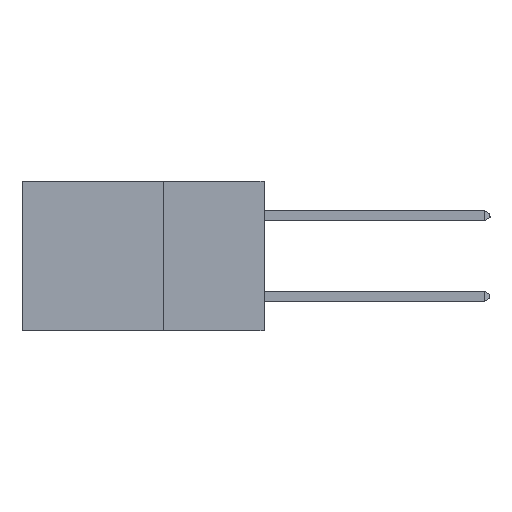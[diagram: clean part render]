
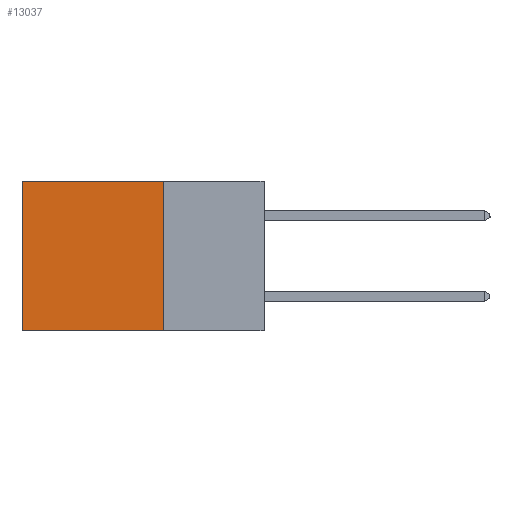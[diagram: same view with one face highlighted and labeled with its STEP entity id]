
A CAD part, left-side view. The second image highlights one B-rep face of the part: STEP entity #13037.
In plain terms, the highlighted planar face has unit normal (-1, 0, 0).
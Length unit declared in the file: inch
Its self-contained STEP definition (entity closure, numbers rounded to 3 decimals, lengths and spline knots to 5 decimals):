
#670 = AXIS2_PLACEMENT_3D ( 'NONE', #2234, #16523, #4302 ) ;
#1079 = CARTESIAN_POINT ( 'NONE',  ( 0.298, 0.6, -0.37 ) ) ;
#1245 = CARTESIAN_POINT ( 'NONE',  ( 0.298, 0.25, 0. ) ) ;
#2234 = CARTESIAN_POINT ( 'NONE',  ( 0.298, 0.25, 0. ) ) ;
#2896 = ORIENTED_EDGE ( 'NONE', *, *, #9898, .T. ) ;
#3037 = EDGE_LOOP ( 'NONE', ( #5047, #13905, #4222, #2896 ) ) ;
#3157 = LINE ( 'NONE', #13598, #13409 ) ;
#4192 = DIRECTION ( 'NONE',  ( 0., 0., -1. ) ) ;
#4195 = CARTESIAN_POINT ( 'NONE',  ( 0.298, 0.25, 0. ) ) ;
#4222 = ORIENTED_EDGE ( 'NONE', *, *, #17154, .F. ) ;
#4302 = DIRECTION ( 'NONE',  ( 0., 0., -1. ) ) ;
#4704 = VERTEX_POINT ( 'NONE', #20211 ) ;
#4715 = LINE ( 'NONE', #16407, #26060 ) ;
#5047 = ORIENTED_EDGE ( 'NONE', *, *, #21842, .T. ) ;
#5475 = LINE ( 'NONE', #1245, #17407 ) ;
#7321 = VECTOR ( 'NONE', #13098, 39.37008 ) ;
#7409 = DIRECTION ( 'NONE',  ( 0., 0., -1. ) ) ;
#8746 = EDGE_CURVE ( 'NONE', #4704, #14799, #3157, .T. ) ;
#9898 = EDGE_CURVE ( 'NONE', #11050, #24743, #23326, .T. ) ;
#11050 = VERTEX_POINT ( 'NONE', #4195 ) ;
#12391 = FACE_OUTER_BOUND ( 'NONE', #3037, .T. ) ;
#13037 = ADVANCED_FACE ( 'NONE', ( #12391 ), #20463, .F. ) ;
#13098 = DIRECTION ( 'NONE',  ( 0., 1., 0. ) ) ;
#13409 = VECTOR ( 'NONE', #13507, 39.37008 ) ;
#13507 = DIRECTION ( 'NONE',  ( 0., 1., 0. ) ) ;
#13598 = CARTESIAN_POINT ( 'NONE',  ( 0.298, 0.25, -0.37 ) ) ;
#13905 = ORIENTED_EDGE ( 'NONE', *, *, #8746, .F. ) ;
#14799 = VERTEX_POINT ( 'NONE', #1079 ) ;
#15453 = CARTESIAN_POINT ( 'NONE',  ( 0.298, 0.6, 0. ) ) ;
#16407 = CARTESIAN_POINT ( 'NONE',  ( 0.298, 0.6, 0. ) ) ;
#16523 = DIRECTION ( 'NONE',  ( 1., 0., 0. ) ) ;
#17154 = EDGE_CURVE ( 'NONE', #11050, #4704, #5475, .T. ) ;
#17407 = VECTOR ( 'NONE', #7409, 39.37008 ) ;
#20211 = CARTESIAN_POINT ( 'NONE',  ( 0.298, 0.25, -0.37 ) ) ;
#20463 = PLANE ( 'NONE',  #670 ) ;
#21842 = EDGE_CURVE ( 'NONE', #24743, #14799, #4715, .T. ) ;
#23146 = CARTESIAN_POINT ( 'NONE',  ( 0.298, 0.25, 0. ) ) ;
#23326 = LINE ( 'NONE', #23146, #7321 ) ;
#24743 = VERTEX_POINT ( 'NONE', #15453 ) ;
#26060 = VECTOR ( 'NONE', #4192, 39.37008 ) ;
